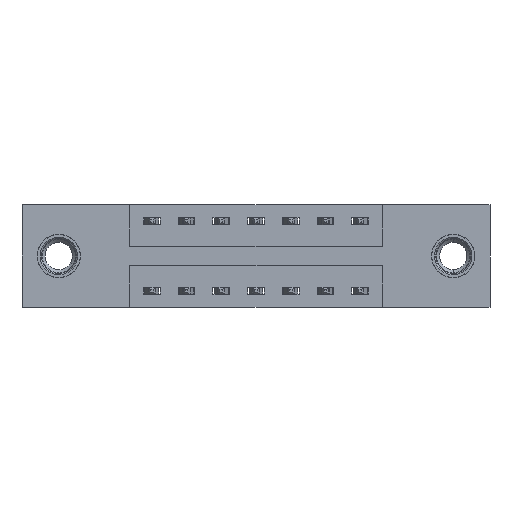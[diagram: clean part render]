
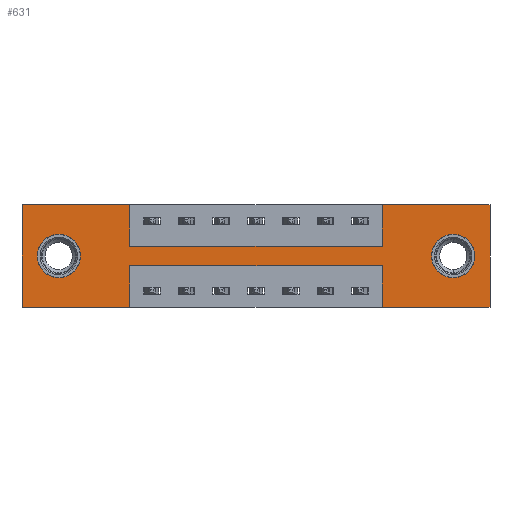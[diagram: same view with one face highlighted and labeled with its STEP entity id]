
A CAD part, front view. The second image highlights one B-rep face of the part: STEP entity #631.
In plain terms, the highlighted planar face has unit normal (0, -1, 0).
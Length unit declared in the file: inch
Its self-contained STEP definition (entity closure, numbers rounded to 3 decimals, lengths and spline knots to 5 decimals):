
#84 = EDGE_CURVE ( 'NONE', #1385, #1068, #282, .T. ) ;
#103 = DIRECTION ( 'NONE',  ( 0., 1., 0. ) ) ;
#209 = EDGE_CURVE ( 'NONE', #1179, #7324, #8699, .T. ) ;
#229 = EDGE_CURVE ( 'NONE', #6393, #916, #10214, .T. ) ;
#263 = ORIENTED_EDGE ( 'NONE', *, *, #1877, .F. ) ;
#265 = EDGE_CURVE ( 'NONE', #10261, #5049, #9758, .T. ) ;
#282 = CIRCLE ( 'NONE', #5104, 0.078 ) ;
#286 = CARTESIAN_POINT ( 'NONE',  ( 0., 0., 0. ) ) ;
#374 = CARTESIAN_POINT ( 'NONE',  ( 0., 0., 0. ) ) ;
#575 = EDGE_CURVE ( 'NONE', #916, #10261, #2899, .T. ) ;
#631 = ADVANCED_FACE ( 'NONE', ( #9850, #3765, #7828 ), #3017, .T. ) ;
#798 = CARTESIAN_POINT ( 'NONE',  ( 1.5525, 0., -0.185 ) ) ;
#865 = CARTESIAN_POINT ( 'NONE',  ( 0.1325, 0., -0.185 ) ) ;
#916 = VERTEX_POINT ( 'NONE', #2787 ) ;
#1031 = VERTEX_POINT ( 'NONE', #9076 ) ;
#1068 = VERTEX_POINT ( 'NONE', #10166 ) ;
#1179 = VERTEX_POINT ( 'NONE', #6414 ) ;
#1194 = DIRECTION ( 'NONE',  ( -1., 0., 0. ) ) ;
#1242 = VECTOR ( 'NONE', #4625, 39.37008 ) ;
#1305 = CARTESIAN_POINT ( 'NONE',  ( 0., 0., -0.37 ) ) ;
#1385 = VERTEX_POINT ( 'NONE', #3522 ) ;
#1427 = VERTEX_POINT ( 'NONE', #8440 ) ;
#1448 = EDGE_CURVE ( 'NONE', #7098, #6393, #4499, .T. ) ;
#1499 = CARTESIAN_POINT ( 'NONE',  ( 0.3875, 0., -0.15 ) ) ;
#1546 = EDGE_CURVE ( 'NONE', #1031, #1179, #4367, .T. ) ;
#1555 = LINE ( 'NONE', #6286, #1242 ) ;
#1751 = DIRECTION ( 'NONE',  ( 0., 0., -1. ) ) ;
#1816 = DIRECTION ( 'NONE',  ( 0., 0., 1. ) ) ;
#1877 = EDGE_CURVE ( 'NONE', #7324, #4016, #1555, .T. ) ;
#1928 = EDGE_LOOP ( 'NONE', ( #9632, #9426 ) ) ;
#2019 = EDGE_CURVE ( 'NONE', #3721, #1031, #4364, .T. ) ;
#2392 = AXIS2_PLACEMENT_3D ( 'NONE', #798, #6630, #1751 ) ;
#2438 = EDGE_LOOP ( 'NONE', ( #9352, #10353, #8078, #9257, #7702, #263, #5082, #7974, #7670, #4528, #4192, #9976 ) ) ;
#2519 = EDGE_CURVE ( 'NONE', #5049, #3721, #3090, .T. ) ;
#2536 = EDGE_CURVE ( 'NONE', #8111, #3374, #5041, .T. ) ;
#2787 = CARTESIAN_POINT ( 'NONE',  ( 0.3875, 0., -0.37 ) ) ;
#2899 = LINE ( 'NONE', #9298, #4836 ) ;
#3017 = PLANE ( 'NONE',  #9629 ) ;
#3090 = LINE ( 'NONE', #374, #7403 ) ;
#3104 = VECTOR ( 'NONE', #7949, 39.37008 ) ;
#3233 = VECTOR ( 'NONE', #9544, 39.37008 ) ;
#3269 = CARTESIAN_POINT ( 'NONE',  ( 0.3875, 0., 0. ) ) ;
#3283 = EDGE_CURVE ( 'NONE', #1427, #5591, #4332, .T. ) ;
#3329 = EDGE_LOOP ( 'NONE', ( #9920, #9300 ) ) ;
#3374 = VERTEX_POINT ( 'NONE', #8329 ) ;
#3407 = VECTOR ( 'NONE', #10119, 39.37008 ) ;
#3522 = CARTESIAN_POINT ( 'NONE',  ( 1.5525, 0., -0.107 ) ) ;
#3721 = VERTEX_POINT ( 'NONE', #3269 ) ;
#3765 = FACE_BOUND ( 'NONE', #3329, .T. ) ;
#3924 = VECTOR ( 'NONE', #4597, 39.37008 ) ;
#4016 = VERTEX_POINT ( 'NONE', #6842 ) ;
#4192 = ORIENTED_EDGE ( 'NONE', *, *, #265, .F. ) ;
#4332 = CIRCLE ( 'NONE', #7523, 0.078 ) ;
#4364 = LINE ( 'NONE', #4859, #10158 ) ;
#4367 = LINE ( 'NONE', #1499, #3233 ) ;
#4370 = DIRECTION ( 'NONE',  ( 0., 0., 1. ) ) ;
#4469 = DIRECTION ( 'NONE',  ( -1., 0., 0. ) ) ;
#4499 = LINE ( 'NONE', #6202, #8515 ) ;
#4528 = ORIENTED_EDGE ( 'NONE', *, *, #2519, .F. ) ;
#4558 = CARTESIAN_POINT ( 'NONE',  ( 1.2975, 0., 0. ) ) ;
#4597 = DIRECTION ( 'NONE',  ( 0., 0., -1. ) ) ;
#4625 = DIRECTION ( 'NONE',  ( 1., 0., 0. ) ) ;
#4665 = DIRECTION ( 'NONE',  ( 0., -1., 0. ) ) ;
#4818 = DIRECTION ( 'NONE',  ( 0., 1., 0. ) ) ;
#4836 = VECTOR ( 'NONE', #4469, 39.37008 ) ;
#4859 = CARTESIAN_POINT ( 'NONE',  ( 0.3875, 0., 0. ) ) ;
#5041 = LINE ( 'NONE', #5520, #9006 ) ;
#5049 = VERTEX_POINT ( 'NONE', #286 ) ;
#5082 = ORIENTED_EDGE ( 'NONE', *, *, #209, .F. ) ;
#5091 = CARTESIAN_POINT ( 'NONE',  ( 0.1325, 0., -0.263 ) ) ;
#5104 = AXIS2_PLACEMENT_3D ( 'NONE', #5227, #103, #6057 ) ;
#5227 = CARTESIAN_POINT ( 'NONE',  ( 1.5525, 0., -0.185 ) ) ;
#5422 = CARTESIAN_POINT ( 'NONE',  ( 1.2975, 0., -0.22 ) ) ;
#5461 = CIRCLE ( 'NONE', #2392, 0.078 ) ;
#5520 = CARTESIAN_POINT ( 'NONE',  ( 0., 0., -0.37 ) ) ;
#5591 = VERTEX_POINT ( 'NONE', #5091 ) ;
#5684 = DIRECTION ( 'NONE',  ( 0., 0., -1. ) ) ;
#6033 = EDGE_CURVE ( 'NONE', #5591, #1427, #8298, .T. ) ;
#6057 = DIRECTION ( 'NONE',  ( 0., 0., -1. ) ) ;
#6202 = CARTESIAN_POINT ( 'NONE',  ( 0.3875, 0., -0.22 ) ) ;
#6286 = CARTESIAN_POINT ( 'NONE',  ( 0., 0., 0. ) ) ;
#6308 = DIRECTION ( 'NONE',  ( 1., 0., 0. ) ) ;
#6341 = DIRECTION ( 'NONE',  ( -1., 0., 0. ) ) ;
#6393 = VERTEX_POINT ( 'NONE', #7465 ) ;
#6414 = CARTESIAN_POINT ( 'NONE',  ( 1.2975, 0., -0.15 ) ) ;
#6451 = CARTESIAN_POINT ( 'NONE',  ( 1.2975, 0., 0. ) ) ;
#6630 = DIRECTION ( 'NONE',  ( 0., 1., 0. ) ) ;
#6685 = DIRECTION ( 'NONE',  ( 0., 1., 0. ) ) ;
#6816 = CARTESIAN_POINT ( 'NONE',  ( 1.2975, 0., -0.37 ) ) ;
#6842 = CARTESIAN_POINT ( 'NONE',  ( 1.685, 0., 0. ) ) ;
#7098 = VERTEX_POINT ( 'NONE', #5422 ) ;
#7324 = VERTEX_POINT ( 'NONE', #6451 ) ;
#7403 = VECTOR ( 'NONE', #6308, 39.37008 ) ;
#7434 = VECTOR ( 'NONE', #4370, 39.37008 ) ;
#7465 = CARTESIAN_POINT ( 'NONE',  ( 0.3875, 0., -0.22 ) ) ;
#7503 = EDGE_CURVE ( 'NONE', #1068, #1385, #5461, .T. ) ;
#7520 = CARTESIAN_POINT ( 'NONE',  ( 0., 0., -0.37 ) ) ;
#7523 = AXIS2_PLACEMENT_3D ( 'NONE', #865, #6685, #1816 ) ;
#7670 = ORIENTED_EDGE ( 'NONE', *, *, #2019, .F. ) ;
#7702 = ORIENTED_EDGE ( 'NONE', *, *, #9542, .F. ) ;
#7767 = DIRECTION ( 'NONE',  ( 0., 0., 1. ) ) ;
#7828 = FACE_OUTER_BOUND ( 'NONE', #2438, .T. ) ;
#7831 = CARTESIAN_POINT ( 'NONE',  ( 0., 0., 0. ) ) ;
#7949 = DIRECTION ( 'NONE',  ( 0., 0., -1. ) ) ;
#7974 = ORIENTED_EDGE ( 'NONE', *, *, #1546, .F. ) ;
#8043 = CARTESIAN_POINT ( 'NONE',  ( 1.685, 0., -0.37 ) ) ;
#8078 = ORIENTED_EDGE ( 'NONE', *, *, #8263, .F. ) ;
#8111 = VERTEX_POINT ( 'NONE', #8043 ) ;
#8263 = EDGE_CURVE ( 'NONE', #3374, #7098, #9721, .T. ) ;
#8298 = CIRCLE ( 'NONE', #10235, 0.078 ) ;
#8329 = CARTESIAN_POINT ( 'NONE',  ( 1.2975, 0., -0.37 ) ) ;
#8440 = CARTESIAN_POINT ( 'NONE',  ( 0.1325, 0., -0.107 ) ) ;
#8515 = VECTOR ( 'NONE', #1194, 39.37008 ) ;
#8572 = CARTESIAN_POINT ( 'NONE',  ( 0.3875, 0., -0.37 ) ) ;
#8699 = LINE ( 'NONE', #4558, #10438 ) ;
#9006 = VECTOR ( 'NONE', #6341, 39.37008 ) ;
#9076 = CARTESIAN_POINT ( 'NONE',  ( 0.3875, 0., -0.15 ) ) ;
#9257 = ORIENTED_EDGE ( 'NONE', *, *, #2536, .F. ) ;
#9298 = CARTESIAN_POINT ( 'NONE',  ( 0., 0., -0.37 ) ) ;
#9300 = ORIENTED_EDGE ( 'NONE', *, *, #6033, .T. ) ;
#9352 = ORIENTED_EDGE ( 'NONE', *, *, #229, .F. ) ;
#9426 = ORIENTED_EDGE ( 'NONE', *, *, #7503, .T. ) ;
#9532 = CARTESIAN_POINT ( 'NONE',  ( 0.1325, 0., -0.185 ) ) ;
#9542 = EDGE_CURVE ( 'NONE', #4016, #8111, #9704, .T. ) ;
#9544 = DIRECTION ( 'NONE',  ( 1., 0., 0. ) ) ;
#9629 = AXIS2_PLACEMENT_3D ( 'NONE', #1305, #4665, #10148 ) ;
#9632 = ORIENTED_EDGE ( 'NONE', *, *, #84, .T. ) ;
#9704 = LINE ( 'NONE', #10205, #3104 ) ;
#9721 = LINE ( 'NONE', #6816, #7434 ) ;
#9758 = LINE ( 'NONE', #7831, #3407 ) ;
#9850 = FACE_BOUND ( 'NONE', #1928, .T. ) ;
#9920 = ORIENTED_EDGE ( 'NONE', *, *, #3283, .T. ) ;
#9976 = ORIENTED_EDGE ( 'NONE', *, *, #575, .F. ) ;
#10119 = DIRECTION ( 'NONE',  ( 0., 0., 1. ) ) ;
#10148 = DIRECTION ( 'NONE',  ( 0., 0., -1. ) ) ;
#10158 = VECTOR ( 'NONE', #5684, 39.37008 ) ;
#10166 = CARTESIAN_POINT ( 'NONE',  ( 1.5525, 0., -0.263 ) ) ;
#10205 = CARTESIAN_POINT ( 'NONE',  ( 1.685, 0., 0. ) ) ;
#10214 = LINE ( 'NONE', #8572, #3924 ) ;
#10235 = AXIS2_PLACEMENT_3D ( 'NONE', #9532, #4818, #10269 ) ;
#10261 = VERTEX_POINT ( 'NONE', #7520 ) ;
#10269 = DIRECTION ( 'NONE',  ( 0., 0., 1. ) ) ;
#10353 = ORIENTED_EDGE ( 'NONE', *, *, #1448, .F. ) ;
#10438 = VECTOR ( 'NONE', #7767, 39.37008 ) ;
